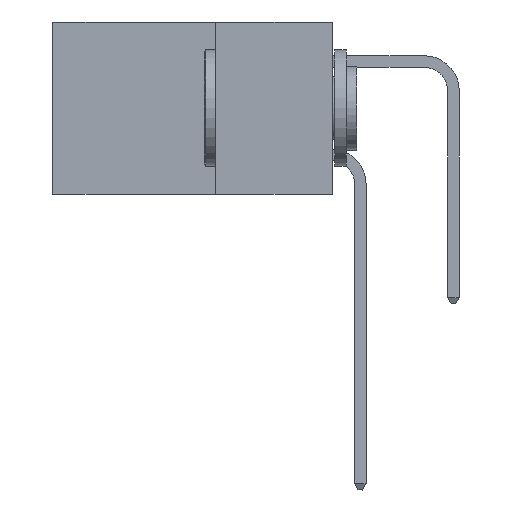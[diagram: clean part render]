
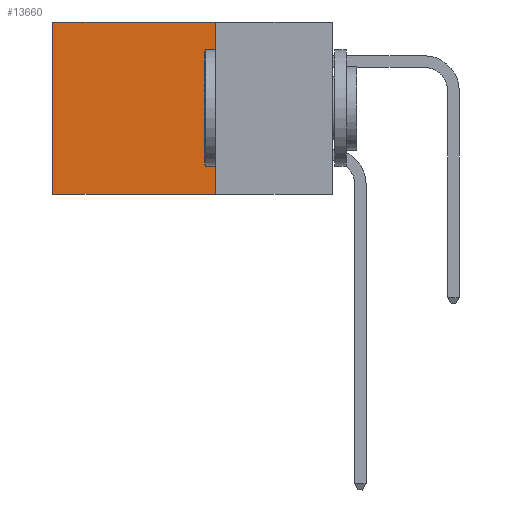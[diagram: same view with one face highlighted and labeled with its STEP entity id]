
A CAD part, left-side view. The second image highlights one B-rep face of the part: STEP entity #13660.
In plain terms, the highlighted planar face has unit normal (-1, 0, 0).
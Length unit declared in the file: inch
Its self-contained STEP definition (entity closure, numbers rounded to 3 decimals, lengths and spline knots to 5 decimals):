
#1057 = CARTESIAN_POINT ( 'NONE',  ( 0.2615, 0.6, -0.37 ) ) ;
#1247 = VECTOR ( 'NONE', #14202, 39.37008 ) ;
#1377 = CARTESIAN_POINT ( 'NONE',  ( 0.2615, 0.25, -0.37 ) ) ;
#2091 = CARTESIAN_POINT ( 'NONE',  ( 0.2615, 0.6, 0. ) ) ;
#3121 = VERTEX_POINT ( 'NONE', #1057 ) ;
#3148 = VERTEX_POINT ( 'NONE', #2091 ) ;
#4044 = LINE ( 'NONE', #15528, #17527 ) ;
#4780 = ORIENTED_EDGE ( 'NONE', *, *, #17590, .T. ) ;
#5573 = DIRECTION ( 'NONE',  ( 0., 1., 0. ) ) ;
#6241 = FACE_OUTER_BOUND ( 'NONE', #12893, .T. ) ;
#6666 = LINE ( 'NONE', #12438, #16405 ) ;
#7783 = ORIENTED_EDGE ( 'NONE', *, *, #13039, .F. ) ;
#8052 = CARTESIAN_POINT ( 'NONE',  ( 0.2615, 0.25, -0.37 ) ) ;
#8308 = VERTEX_POINT ( 'NONE', #1377 ) ;
#8415 = LINE ( 'NONE', #14370, #1247 ) ;
#8522 = ORIENTED_EDGE ( 'NONE', *, *, #11283, .F. ) ;
#9027 = VECTOR ( 'NONE', #14251, 39.37008 ) ;
#9294 = PLANE ( 'NONE',  #15193 ) ;
#10086 = CARTESIAN_POINT ( 'NONE',  ( 0.2615, 0.25, 0. ) ) ;
#10991 = DIRECTION ( 'NONE',  ( 1., 0., 0. ) ) ;
#11283 = EDGE_CURVE ( 'NONE', #8308, #3121, #4044, .T. ) ;
#11310 = EDGE_CURVE ( 'NONE', #3148, #3121, #8415, .T. ) ;
#11618 = ORIENTED_EDGE ( 'NONE', *, *, #11310, .T. ) ;
#12304 = DIRECTION ( 'NONE',  ( 0., 0., -1. ) ) ;
#12438 = CARTESIAN_POINT ( 'NONE',  ( 0.2615, 0.25, -0.37 ) ) ;
#12505 = CARTESIAN_POINT ( 'NONE',  ( 0.2615, 0.25, 0. ) ) ;
#12826 = LINE ( 'NONE', #10086, #9027 ) ;
#12893 = EDGE_LOOP ( 'NONE', ( #11618, #8522, #7783, #4780 ) ) ;
#13039 = EDGE_CURVE ( 'NONE', #13809, #8308, #6666, .T. ) ;
#13660 = ADVANCED_FACE ( 'NONE', ( #6241 ), #9294, .F. ) ;
#13809 = VERTEX_POINT ( 'NONE', #12505 ) ;
#14202 = DIRECTION ( 'NONE',  ( 0., 0., -1. ) ) ;
#14251 = DIRECTION ( 'NONE',  ( 0., 1., 0. ) ) ;
#14370 = CARTESIAN_POINT ( 'NONE',  ( 0.2615, 0.6, -0.37 ) ) ;
#15193 = AXIS2_PLACEMENT_3D ( 'NONE', #8052, #10991, #12304 ) ;
#15528 = CARTESIAN_POINT ( 'NONE',  ( 0.2615, 0.25, -0.37 ) ) ;
#16405 = VECTOR ( 'NONE', #18207, 39.37008 ) ;
#17527 = VECTOR ( 'NONE', #5573, 39.37008 ) ;
#17590 = EDGE_CURVE ( 'NONE', #13809, #3148, #12826, .T. ) ;
#18207 = DIRECTION ( 'NONE',  ( 0., 0., -1. ) ) ;
